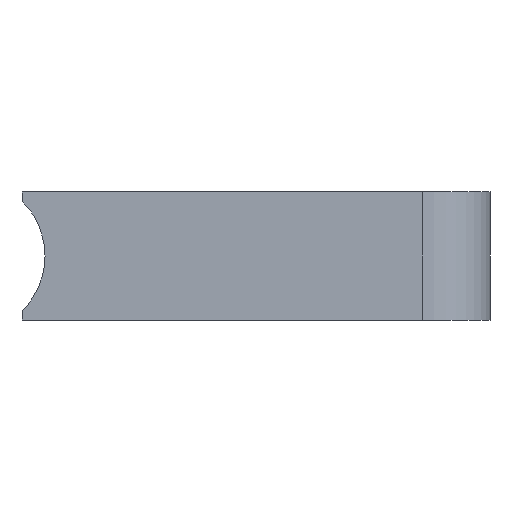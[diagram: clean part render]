
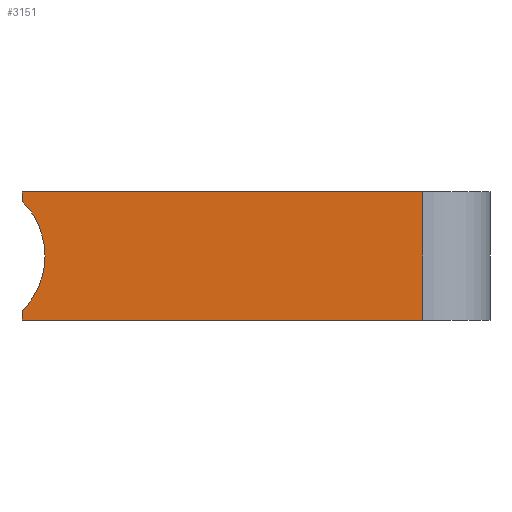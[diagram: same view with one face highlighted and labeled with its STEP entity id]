
A CAD part, left-side view. The second image highlights one B-rep face of the part: STEP entity #3151.
In plain terms, the highlighted planar face has unit normal (-1, 0, 0).
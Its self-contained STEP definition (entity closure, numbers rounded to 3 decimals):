
#769 = CYLINDRICAL_SURFACE('',#770,4.875);
#770 = AXIS2_PLACEMENT_3D('',#771,#772,#773);
#771 = CARTESIAN_POINT('',(-13.686,28.517,4.));
#772 = DIRECTION('',(-0.996,0.087,
    0.));
#773 = DIRECTION('',(-0.087,-0.996,
    0.));
#802 = PLANE('',#803);
#803 = AXIS2_PLACEMENT_3D('',#804,#805,#806);
#804 = CARTESIAN_POINT('',(-13.,25.,8.));
#805 = DIRECTION('',(-0.087,-0.996,0.));
#806 = DIRECTION('',(0.996,-0.087,0.));
#883 = PLANE('',#884);
#884 = AXIS2_PLACEMENT_3D('',#885,#886,#887);
#885 = CARTESIAN_POINT('',(-13.,25.,8.));
#886 = DIRECTION('',(-0.087,-0.996,0.));
#887 = DIRECTION('',(0.996,-0.087,0.));
#909 = CYLINDRICAL_SURFACE('',#910,4.875);
#910 = AXIS2_PLACEMENT_3D('',#911,#912,#913);
#911 = CARTESIAN_POINT('',(-13.686,28.517,4.));
#912 = DIRECTION('',(-0.996,0.087,
    0.));
#913 = DIRECTION('',(-0.087,-0.996,
    0.));
#1127 = PLANE('',#1128);
#1128 = AXIS2_PLACEMENT_3D('',#1129,#1130,#1131);
#1129 = CARTESIAN_POINT('',(0.,0.,0.));
#1130 = DIRECTION('',(0.,0.,1.));
#1131 = DIRECTION('',(1.,0.,0.));
#1698 = PLANE('',#1699);
#1699 = AXIS2_PLACEMENT_3D('',#1700,#1701,#1702);
#1700 = CARTESIAN_POINT('',(0.,0.,8.));
#1701 = DIRECTION('',(0.,0.,1.));
#1702 = DIRECTION('',(1.,0.,0.));
#1954 = VERTEX_POINT('',#1955);
#1955 = CARTESIAN_POINT('',(-13.,25.,0.55));
#1976 = VERTEX_POINT('',#1977);
#1977 = CARTESIAN_POINT('',(-13.,23.564,4.));
#1998 = EDGE_CURVE('',#1954,#1976,#1999,.T.);
#1999 = SURFACE_CURVE('',#2000,(#2005,#2018),.PCURVE_S1.);
#2000 = ELLIPSE('',#2001,4.893,4.875);
#2001 = AXIS2_PLACEMENT_3D('',#2002,#2003,#2004);
#2002 = CARTESIAN_POINT('',(-13.,28.458,4.));
#2003 = DIRECTION('',(-1.,0.,0.));
#2004 = DIRECTION('',(0.,1.,0.));
#2005 = PCURVE('',#769,#2006);
#2006 = DEFINITIONAL_REPRESENTATION('',(#2007),#2017);
#2007 = B_SPLINE_CURVE_WITH_KNOTS('',8,(#2008,#2009,#2010,#2011,#2012,
    #2013,#2014,#2015,#2016),.UNSPECIFIED.,.F.,.F.,(9,9),(1.768
    ,4.515),.PIECEWISE_BEZIER_KNOTS.);
#2008 = CARTESIAN_POINT('',(4.909,-0.771));
#2009 = CARTESIAN_POINT('',(5.253,-0.914));
#2010 = CARTESIAN_POINT('',(5.596,-1.046));
#2011 = CARTESIAN_POINT('',(5.94,-1.141));
#2012 = CARTESIAN_POINT('',(6.283,-1.176));
#2013 = CARTESIAN_POINT('',(6.627,-1.141));
#2014 = CARTESIAN_POINT('',(6.97,-1.046));
#2015 = CARTESIAN_POINT('',(7.314,-0.914));
#2016 = CARTESIAN_POINT('',(7.657,-0.771));
#2017 = ( GEOMETRIC_REPRESENTATION_CONTEXT(2) 
PARAMETRIC_REPRESENTATION_CONTEXT() REPRESENTATION_CONTEXT('2D SPACE',''
  ) );
#2018 = PCURVE('',#2019,#2024);
#2019 = PLANE('',#2020);
#2020 = AXIS2_PLACEMENT_3D('',#2021,#2022,#2023);
#2021 = CARTESIAN_POINT('',(-13.,0.,0.));
#2022 = DIRECTION('',(-1.,0.,0.));
#2023 = DIRECTION('',(0.,1.,0.));
#2024 = DEFINITIONAL_REPRESENTATION('',(#2025),#2029);
#2025 = ELLIPSE('',#2026,4.893,4.875);
#2026 = AXIS2_PLACEMENT_2D('',#2027,#2028);
#2027 = CARTESIAN_POINT('',(28.458,-4.));
#2028 = DIRECTION('',(1.,0.));
#2029 = ( GEOMETRIC_REPRESENTATION_CONTEXT(2) 
PARAMETRIC_REPRESENTATION_CONTEXT() REPRESENTATION_CONTEXT('2D SPACE',''
  ) );
#2037 = VERTEX_POINT('',#2038);
#2038 = CARTESIAN_POINT('',(-13.,25.,7.45));
#2057 = EDGE_CURVE('',#1976,#2037,#2058,.T.);
#2058 = SURFACE_CURVE('',#2059,(#2064,#2077),.PCURVE_S1.);
#2059 = ELLIPSE('',#2060,4.893,4.875);
#2060 = AXIS2_PLACEMENT_3D('',#2061,#2062,#2063);
#2061 = CARTESIAN_POINT('',(-13.,28.458,4.));
#2062 = DIRECTION('',(-1.,0.,0.));
#2063 = DIRECTION('',(0.,1.,0.));
#2064 = PCURVE('',#909,#2065);
#2065 = DEFINITIONAL_REPRESENTATION('',(#2066),#2076);
#2066 = B_SPLINE_CURVE_WITH_KNOTS('',8,(#2067,#2068,#2069,#2070,#2071,
    #2072,#2073,#2074,#2075),.UNSPECIFIED.,.F.,.F.,(9,9),(1.768
    ,4.515),.PIECEWISE_BEZIER_KNOTS.);
#2067 = CARTESIAN_POINT('',(-1.374,-0.771));
#2068 = CARTESIAN_POINT('',(-1.03,-0.914));
#2069 = CARTESIAN_POINT('',(-0.687,-1.046));
#2070 = CARTESIAN_POINT('',(-0.343,-1.141));
#2071 = CARTESIAN_POINT('',(0.,-1.176));
#2072 = CARTESIAN_POINT('',(0.343,-1.141));
#2073 = CARTESIAN_POINT('',(0.687,-1.046));
#2074 = CARTESIAN_POINT('',(1.03,-0.914));
#2075 = CARTESIAN_POINT('',(1.374,-0.771));
#2076 = ( GEOMETRIC_REPRESENTATION_CONTEXT(2) 
PARAMETRIC_REPRESENTATION_CONTEXT() REPRESENTATION_CONTEXT('2D SPACE',''
  ) );
#2077 = PCURVE('',#2019,#2078);
#2078 = DEFINITIONAL_REPRESENTATION('',(#2079),#2083);
#2079 = ELLIPSE('',#2080,4.893,4.875);
#2080 = AXIS2_PLACEMENT_2D('',#2081,#2082);
#2081 = CARTESIAN_POINT('',(28.458,-4.));
#2082 = DIRECTION('',(1.,0.));
#2083 = ( GEOMETRIC_REPRESENTATION_CONTEXT(2) 
PARAMETRIC_REPRESENTATION_CONTEXT() REPRESENTATION_CONTEXT('2D SPACE',''
  ) );
#2159 = VERTEX_POINT('',#2160);
#2160 = CARTESIAN_POINT('',(-13.,25.,8.));
#2181 = EDGE_CURVE('',#2037,#2159,#2182,.T.);
#2182 = SURFACE_CURVE('',#2183,(#2187,#2194),.PCURVE_S1.);
#2183 = LINE('',#2184,#2185);
#2184 = CARTESIAN_POINT('',(-13.,25.,0.));
#2185 = VECTOR('',#2186,1.);
#2186 = DIRECTION('',(0.,0.,1.));
#2187 = PCURVE('',#883,#2188);
#2188 = DEFINITIONAL_REPRESENTATION('',(#2189),#2193);
#2189 = LINE('',#2190,#2191);
#2190 = CARTESIAN_POINT('',(0.,-8.));
#2191 = VECTOR('',#2192,1.);
#2192 = DIRECTION('',(0.,1.));
#2193 = ( GEOMETRIC_REPRESENTATION_CONTEXT(2) 
PARAMETRIC_REPRESENTATION_CONTEXT() REPRESENTATION_CONTEXT('2D SPACE',''
  ) );
#2194 = PCURVE('',#2019,#2195);
#2195 = DEFINITIONAL_REPRESENTATION('',(#2196),#2200);
#2196 = LINE('',#2197,#2198);
#2197 = CARTESIAN_POINT('',(25.,0.));
#2198 = VECTOR('',#2199,1.);
#2199 = DIRECTION('',(0.,-1.));
#2200 = ( GEOMETRIC_REPRESENTATION_CONTEXT(2) 
PARAMETRIC_REPRESENTATION_CONTEXT() REPRESENTATION_CONTEXT('2D SPACE',''
  ) );
#2327 = EDGE_CURVE('',#2328,#1954,#2330,.T.);
#2328 = VERTEX_POINT('',#2329);
#2329 = CARTESIAN_POINT('',(-13.,25.,0.));
#2330 = SURFACE_CURVE('',#2331,(#2335,#2342),.PCURVE_S1.);
#2331 = LINE('',#2332,#2333);
#2332 = CARTESIAN_POINT('',(-13.,25.,0.));
#2333 = VECTOR('',#2334,1.);
#2334 = DIRECTION('',(0.,0.,1.));
#2335 = PCURVE('',#802,#2336);
#2336 = DEFINITIONAL_REPRESENTATION('',(#2337),#2341);
#2337 = LINE('',#2338,#2339);
#2338 = CARTESIAN_POINT('',(0.,-8.));
#2339 = VECTOR('',#2340,1.);
#2340 = DIRECTION('',(0.,1.));
#2341 = ( GEOMETRIC_REPRESENTATION_CONTEXT(2) 
PARAMETRIC_REPRESENTATION_CONTEXT() REPRESENTATION_CONTEXT('2D SPACE',''
  ) );
#2342 = PCURVE('',#2019,#2343);
#2343 = DEFINITIONAL_REPRESENTATION('',(#2344),#2348);
#2344 = LINE('',#2345,#2346);
#2345 = CARTESIAN_POINT('',(25.,0.));
#2346 = VECTOR('',#2347,1.);
#2347 = DIRECTION('',(0.,-1.));
#2348 = ( GEOMETRIC_REPRESENTATION_CONTEXT(2) 
PARAMETRIC_REPRESENTATION_CONTEXT() REPRESENTATION_CONTEXT('2D SPACE',''
  ) );
#2539 = EDGE_CURVE('',#2540,#2328,#2542,.T.);
#2540 = VERTEX_POINT('',#2541);
#2541 = CARTESIAN_POINT('',(-13.,0.,0.));
#2542 = SURFACE_CURVE('',#2543,(#2547,#2554),.PCURVE_S1.);
#2543 = LINE('',#2544,#2545);
#2544 = CARTESIAN_POINT('',(-13.,0.,0.));
#2545 = VECTOR('',#2546,1.);
#2546 = DIRECTION('',(0.,1.,0.));
#2547 = PCURVE('',#1127,#2548);
#2548 = DEFINITIONAL_REPRESENTATION('',(#2549),#2553);
#2549 = LINE('',#2550,#2551);
#2550 = CARTESIAN_POINT('',(-13.,0.));
#2551 = VECTOR('',#2552,1.);
#2552 = DIRECTION('',(0.,1.));
#2553 = ( GEOMETRIC_REPRESENTATION_CONTEXT(2) 
PARAMETRIC_REPRESENTATION_CONTEXT() REPRESENTATION_CONTEXT('2D SPACE',''
  ) );
#2554 = PCURVE('',#2019,#2555);
#2555 = DEFINITIONAL_REPRESENTATION('',(#2556),#2560);
#2556 = LINE('',#2557,#2558);
#2557 = CARTESIAN_POINT('',(0.,0.));
#2558 = VECTOR('',#2559,1.);
#2559 = DIRECTION('',(1.,0.));
#2560 = ( GEOMETRIC_REPRESENTATION_CONTEXT(2) 
PARAMETRIC_REPRESENTATION_CONTEXT() REPRESENTATION_CONTEXT('2D SPACE',''
  ) );
#2576 = PLANE('',#2577);
#2577 = AXIS2_PLACEMENT_3D('',#2578,#2579,#2580);
#2578 = CARTESIAN_POINT('',(0.,0.,0.));
#2579 = DIRECTION('',(0.,-1.,0.));
#2580 = DIRECTION('',(-1.,0.,0.));
#2913 = VERTEX_POINT('',#2914);
#2914 = CARTESIAN_POINT('',(-13.,0.,8.));
#2937 = EDGE_CURVE('',#2913,#2159,#2938,.T.);
#2938 = SURFACE_CURVE('',#2939,(#2943,#2950),.PCURVE_S1.);
#2939 = LINE('',#2940,#2941);
#2940 = CARTESIAN_POINT('',(-13.,0.,8.));
#2941 = VECTOR('',#2942,1.);
#2942 = DIRECTION('',(0.,1.,0.));
#2943 = PCURVE('',#1698,#2944);
#2944 = DEFINITIONAL_REPRESENTATION('',(#2945),#2949);
#2945 = LINE('',#2946,#2947);
#2946 = CARTESIAN_POINT('',(-13.,0.));
#2947 = VECTOR('',#2948,1.);
#2948 = DIRECTION('',(0.,1.));
#2949 = ( GEOMETRIC_REPRESENTATION_CONTEXT(2) 
PARAMETRIC_REPRESENTATION_CONTEXT() REPRESENTATION_CONTEXT('2D SPACE',''
  ) );
#2950 = PCURVE('',#2019,#2951);
#2951 = DEFINITIONAL_REPRESENTATION('',(#2952),#2956);
#2952 = LINE('',#2953,#2954);
#2953 = CARTESIAN_POINT('',(0.,-8.));
#2954 = VECTOR('',#2955,1.);
#2955 = DIRECTION('',(1.,0.));
#2956 = ( GEOMETRIC_REPRESENTATION_CONTEXT(2) 
PARAMETRIC_REPRESENTATION_CONTEXT() REPRESENTATION_CONTEXT('2D SPACE',''
  ) );
#3151 = ADVANCED_FACE('',(#3152),#2019,.T.);
#3152 = FACE_BOUND('',#3153,.T.);
#3153 = EDGE_LOOP('',(#3154,#3155,#3156,#3157,#3178,#3179,#3180));
#3154 = ORIENTED_EDGE('',*,*,#1998,.F.);
#3155 = ORIENTED_EDGE('',*,*,#2327,.F.);
#3156 = ORIENTED_EDGE('',*,*,#2539,.F.);
#3157 = ORIENTED_EDGE('',*,*,#3158,.T.);
#3158 = EDGE_CURVE('',#2540,#2913,#3159,.T.);
#3159 = SURFACE_CURVE('',#3160,(#3164,#3171),.PCURVE_S1.);
#3160 = LINE('',#3161,#3162);
#3161 = CARTESIAN_POINT('',(-13.,0.,0.));
#3162 = VECTOR('',#3163,1.);
#3163 = DIRECTION('',(0.,0.,1.));
#3164 = PCURVE('',#2019,#3165);
#3165 = DEFINITIONAL_REPRESENTATION('',(#3166),#3170);
#3166 = LINE('',#3167,#3168);
#3167 = CARTESIAN_POINT('',(0.,0.));
#3168 = VECTOR('',#3169,1.);
#3169 = DIRECTION('',(0.,-1.));
#3170 = ( GEOMETRIC_REPRESENTATION_CONTEXT(2) 
PARAMETRIC_REPRESENTATION_CONTEXT() REPRESENTATION_CONTEXT('2D SPACE',''
  ) );
#3171 = PCURVE('',#2576,#3172);
#3172 = DEFINITIONAL_REPRESENTATION('',(#3173),#3177);
#3173 = LINE('',#3174,#3175);
#3174 = CARTESIAN_POINT('',(13.,0.));
#3175 = VECTOR('',#3176,1.);
#3176 = DIRECTION('',(0.,-1.));
#3177 = ( GEOMETRIC_REPRESENTATION_CONTEXT(2) 
PARAMETRIC_REPRESENTATION_CONTEXT() REPRESENTATION_CONTEXT('2D SPACE',''
  ) );
#3178 = ORIENTED_EDGE('',*,*,#2937,.T.);
#3179 = ORIENTED_EDGE('',*,*,#2181,.F.);
#3180 = ORIENTED_EDGE('',*,*,#2057,.F.);
